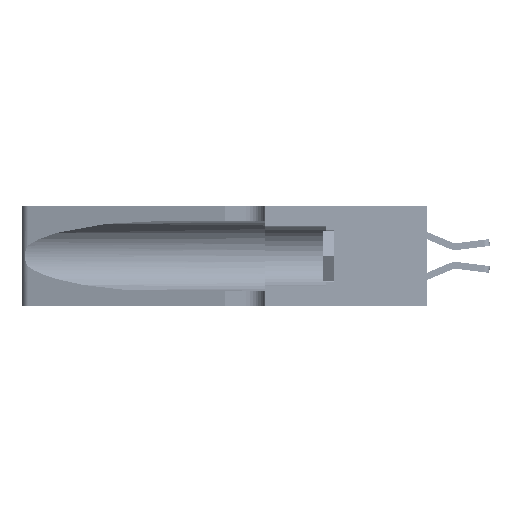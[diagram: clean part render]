
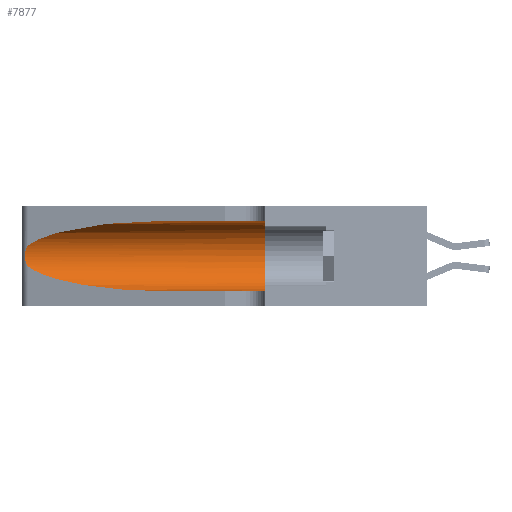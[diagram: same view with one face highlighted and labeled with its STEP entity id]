
A CAD part, left-side view. The second image highlights one B-rep face of the part: STEP entity #7877.
In plain terms, the highlighted cylindrical face has radius 3.308 mm (diameter 6.617 mm), a partial arc.
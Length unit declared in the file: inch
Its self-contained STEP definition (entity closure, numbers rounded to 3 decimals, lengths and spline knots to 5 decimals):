
#414 = VECTOR ( 'NONE', #10336, 39.37008 ) ;
#519 = FACE_OUTER_BOUND ( 'NONE', #22773, .T. ) ;
#1106 = CARTESIAN_POINT ( 'NONE',  ( 0.25555, 1.22994, 0.2215 ) ) ;
#1496 = CARTESIAN_POINT ( 'NONE',  ( 0.25487, 1.22718, 0.14631 ) ) ;
#2382 = ORIENTED_EDGE ( 'NONE', *, *, #37882, .F. ) ;
#3624 = CARTESIAN_POINT ( 'NONE',  ( 0.26017, 1.23833, 0.17102 ) ) ;
#3831 = CARTESIAN_POINT ( 'NONE',  ( 0.2373, 1.15595, 0.08982 ) ) ;
#3834 = CARTESIAN_POINT ( 'NONE',  ( 0.1305, 1.61858, 0.05475 ) ) ;
#3918 = DIRECTION ( 'NONE',  ( 0., 0., -1. ) ) ;
#5566 = AXIS2_PLACEMENT_3D ( 'NONE', #16608, #39509, #13641 ) ;
#6897 = CARTESIAN_POINT ( 'NONE',  ( 0.25856, 1.23593, 0.16098 ) ) ;
#7032 = CARTESIAN_POINT ( 'NONE',  ( 0.25639, 1.23184, 0.21858 ) ) ;
#7145 = EDGE_CURVE ( 'NONE', #26123, #16122, #22884, .T. ) ;
#7877 = ADVANCED_FACE ( 'NONE', ( #519 ), #9660, .F. ) ;
#8150 = CARTESIAN_POINT ( 'NONE',  ( 0.18966, 0.96281, 0.31525 ) ) ;
#8714 = EDGE_CURVE ( 'NONE', #23437, #12949, #28639, .T. ) ;
#8790 = CARTESIAN_POINT ( 'NONE',  ( 0.25487, 1.22718, 0.22369 ) ) ;
#9660 = CYLINDRICAL_SURFACE ( 'NONE', #14943, 0.13025 ) ;
#9813 = EDGE_CURVE ( 'NONE', #16122, #11099, #16637, .T. ) ;
#10119 = CARTESIAN_POINT ( 'NONE',  ( 0.25639, 1.23186, 0.15144 ) ) ;
#10336 = DIRECTION ( 'NONE',  ( 0., -1., 0. ) ) ;
#10629 = VECTOR ( 'NONE', #27680, 39.37008 ) ;
#11099 = VERTEX_POINT ( 'NONE', #22389 ) ;
#11284 = CARTESIAN_POINT ( 'NONE',  ( 0.2373, 1.15595, 0.28018 ) ) ;
#12614 = EDGE_CURVE ( 'NONE', #38040, #11099, #21076, .T. ) ;
#12949 = VERTEX_POINT ( 'NONE', #41783 ) ;
#13641 = DIRECTION ( 'NONE',  ( 0., 0., 1. ) ) ;
#13702 = CARTESIAN_POINT ( 'NONE',  ( 0.26018, 1.23835, 0.19895 ) ) ;
#14943 = AXIS2_PLACEMENT_3D ( 'NONE', #29915, #20063, #3918 ) ;
#15567 = CARTESIAN_POINT ( 'NONE',  ( 0.1305, 0.72297, 0.05475 ) ) ;
#15655 = EDGE_CURVE ( 'NONE', #12949, #26123, #34382, .T. ) ;
#15706 = CARTESIAN_POINT ( 'NONE',  ( 0.1305, 0.35, 0.31525 ) ) ;
#16018 = ORIENTED_EDGE ( 'NONE', *, *, #9813, .T. ) ;
#16122 = VERTEX_POINT ( 'NONE', #15567 ) ;
#16608 = CARTESIAN_POINT ( 'NONE',  ( 0.1305, 0.35, 0.185 ) ) ;
#16637 = LINE ( 'NONE', #3834, #414 ) ;
#17237 = CARTESIAN_POINT ( 'NONE',  ( 0.25854, 1.2359, 0.20912 ) ) ;
#18004 = CARTESIAN_POINT ( 'NONE',  ( 0.1305, 1.61858, 0.31525 ) ) ;
#19288 = ORIENTED_EDGE ( 'NONE', *, *, #15655, .T. ) ;
#20063 = DIRECTION ( 'NONE',  ( 0., -1., 0. ) ) ;
#21076 = CIRCLE ( 'NONE', #5566, 0.13025 ) ;
#22389 = CARTESIAN_POINT ( 'NONE',  ( 0.1305, 0.35, 0.05475 ) ) ;
#22773 = EDGE_LOOP ( 'NONE', ( #32757, #19288, #41546, #16018, #37185, #2382 ) ) ;
#22884 =( BOUNDED_CURVE ( )  B_SPLINE_CURVE ( 3, ( #29416, #3831, #29833, #36367 ),
 .UNSPECIFIED., .F., .F. ) 
 B_SPLINE_CURVE_WITH_KNOTS ( ( 4, 4 ),
 ( 3.44316, 4.71239 ),
 .UNSPECIFIED. ) 
 CURVE ( )  GEOMETRIC_REPRESENTATION_ITEM ( )  RATIONAL_B_SPLINE_CURVE ( ( 1., 0.87, 0.87, 1. ) ) 
 REPRESENTATION_ITEM ( '' )  );
#23326 = CARTESIAN_POINT ( 'NONE',  ( 0.26075, 1.23896, 0.19203 ) ) ;
#23437 = VERTEX_POINT ( 'NONE', #28172 ) ;
#26123 = VERTEX_POINT ( 'NONE', #1496 ) ;
#27680 = DIRECTION ( 'NONE',  ( 0., -1., 0. ) ) ;
#27780 = CARTESIAN_POINT ( 'NONE',  ( 0.1305, 0.72297, 0.31525 ) ) ;
#28172 = CARTESIAN_POINT ( 'NONE',  ( 0.1305, 0.72297, 0.31525 ) ) ;
#28639 =( BOUNDED_CURVE ( )  B_SPLINE_CURVE ( 3, ( #27780, #8150, #11284, #30928 ),
 .UNSPECIFIED., .F., .F. ) 
 B_SPLINE_CURVE_WITH_KNOTS ( ( 4, 4 ),
 ( 1.5708, 2.84003 ),
 .UNSPECIFIED. ) 
 CURVE ( )  GEOMETRIC_REPRESENTATION_ITEM ( )  RATIONAL_B_SPLINE_CURVE ( ( 1., 0.87, 0.87, 1. ) ) 
 REPRESENTATION_ITEM ( '' )  );
#29416 = CARTESIAN_POINT ( 'NONE',  ( 0.25487, 1.22718, 0.14631 ) ) ;
#29629 = CARTESIAN_POINT ( 'NONE',  ( 0.25789, 1.23486, 0.15765 ) ) ;
#29833 = CARTESIAN_POINT ( 'NONE',  ( 0.18966, 0.96281, 0.05475 ) ) ;
#29915 = CARTESIAN_POINT ( 'NONE',  ( 0.1305, 1.61858, 0.185 ) ) ;
#30928 = CARTESIAN_POINT ( 'NONE',  ( 0.25487, 1.22718, 0.22369 ) ) ;
#31049 = LINE ( 'NONE', #18004, #10629 ) ;
#32757 = ORIENTED_EDGE ( 'NONE', *, *, #8714, .T. ) ;
#32885 = CARTESIAN_POINT ( 'NONE',  ( 0.25487, 1.22718, 0.14631 ) ) ;
#34382 = B_SPLINE_CURVE_WITH_KNOTS ( 'NONE', 3,
 ( #8790, #1106, #7032, #36749, #17237, #13702, #23326, #39994, #3624, #6897, #29629, #10119, #36458, #32885 ),
 .UNSPECIFIED., .F., .F.,
 ( 4, 2, 2, 2, 2, 2, 4 ),
 ( 0., 0.00027, 0.00053, 0.00107, 0.0016, 0.00187, 0.00214 ),
 .UNSPECIFIED. ) ;
#36367 = CARTESIAN_POINT ( 'NONE',  ( 0.1305, 0.72297, 0.05475 ) ) ;
#36458 = CARTESIAN_POINT ( 'NONE',  ( 0.25555, 1.22993, 0.14849 ) ) ;
#36749 = CARTESIAN_POINT ( 'NONE',  ( 0.25787, 1.23484, 0.2124 ) ) ;
#37185 = ORIENTED_EDGE ( 'NONE', *, *, #12614, .F. ) ;
#37882 = EDGE_CURVE ( 'NONE', #23437, #38040, #31049, .T. ) ;
#38040 = VERTEX_POINT ( 'NONE', #15706 ) ;
#39509 = DIRECTION ( 'NONE',  ( 0., 1., 0. ) ) ;
#39994 = CARTESIAN_POINT ( 'NONE',  ( 0.26075, 1.23896, 0.178 ) ) ;
#41546 = ORIENTED_EDGE ( 'NONE', *, *, #7145, .T. ) ;
#41783 = CARTESIAN_POINT ( 'NONE',  ( 0.25487, 1.22718, 0.22369 ) ) ;
